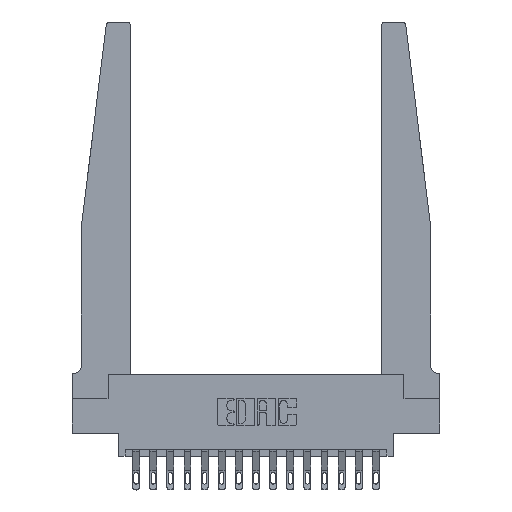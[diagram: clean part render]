
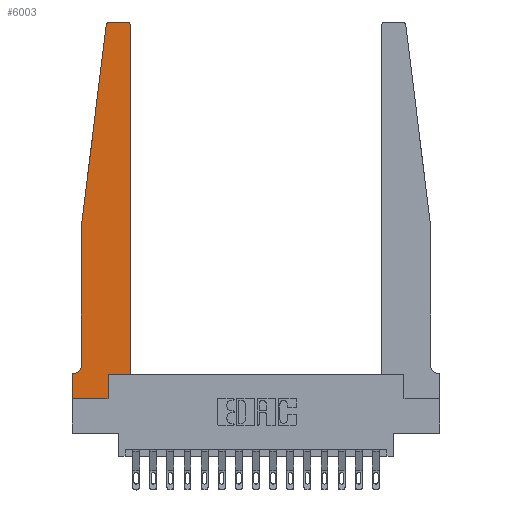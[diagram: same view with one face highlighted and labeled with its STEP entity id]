
A CAD part, top view. The second image highlights one B-rep face of the part: STEP entity #6003.
In plain terms, the highlighted planar face has unit normal (0, 0, 1).
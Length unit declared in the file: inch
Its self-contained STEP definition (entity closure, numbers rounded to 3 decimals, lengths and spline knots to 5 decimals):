
#210 = CARTESIAN_POINT ( 'NONE',  ( 0.425, 0.18, 0.37 ) ) ;
#333 = VECTOR ( 'NONE', #3226, 39.37008 ) ;
#640 = AXIS2_PLACEMENT_3D ( 'NONE', #4934, #15009, #6401 ) ;
#724 = VERTEX_POINT ( 'NONE', #5051 ) ;
#827 = CARTESIAN_POINT ( 'NONE',  ( 0.425, 0.18, 0.37 ) ) ;
#1006 = CARTESIAN_POINT ( 'NONE',  ( 0.27653, 2.75, 0.37 ) ) ;
#1449 = CARTESIAN_POINT ( 'NONE',  ( 0.25, 2.75, 0.37 ) ) ;
#2075 = CARTESIAN_POINT ( 'NONE',  ( 0., 0., 0.37 ) ) ;
#2310 = DIRECTION ( 'NONE',  ( 1., 0., 0. ) ) ;
#2423 = EDGE_CURVE ( 'NONE', #5248, #4190, #13444, .T. ) ;
#2569 = CARTESIAN_POINT ( 'NONE',  ( 0.395, 2.72, 0.37 ) ) ;
#2799 = PLANE ( 'NONE',  #7952 ) ;
#2876 = AXIS2_PLACEMENT_3D ( 'NONE', #2569, #12668, #4031 ) ;
#2906 = LINE ( 'NONE', #6625, #14834 ) ;
#2973 = EDGE_LOOP ( 'NONE', ( #6811, #7140, #7022, #7364, #7803, #7766, #8474, #8508, #8243, #8955, #8969, #13601 ) ) ;
#3065 = LINE ( 'NONE', #827, #10710 ) ;
#3211 = VERTEX_POINT ( 'NONE', #5822 ) ;
#3226 = DIRECTION ( 'NONE',  ( 0., 1., 0. ) ) ;
#3667 = EDGE_CURVE ( 'NONE', #18631, #15239, #2906, .T. ) ;
#3843 = EDGE_CURVE ( 'NONE', #15239, #3211, #15039, .T. ) ;
#4031 = DIRECTION ( 'NONE',  ( 1., 0., 0. ) ) ;
#4035 = CIRCLE ( 'NONE', #640, 0.03 ) ;
#4190 = VERTEX_POINT ( 'NONE', #9826 ) ;
#4252 = DIRECTION ( 'NONE',  ( 1., 0., 0. ) ) ;
#4304 = DIRECTION ( 'NONE',  ( -1., 0., 0. ) ) ;
#4420 = VERTEX_POINT ( 'NONE', #13233 ) ;
#4587 = EDGE_CURVE ( 'NONE', #4783, #18255, #4035, .T. ) ;
#4783 = VERTEX_POINT ( 'NONE', #1006 ) ;
#4934 = CARTESIAN_POINT ( 'NONE',  ( 0.27653, 2.72, 0.37 ) ) ;
#5027 = VERTEX_POINT ( 'NONE', #8942 ) ;
#5051 = CARTESIAN_POINT ( 'NONE',  ( 0.425, 2.72, 0.37 ) ) ;
#5175 = EDGE_CURVE ( 'NONE', #5871, #5248, #10325, .T. ) ;
#5248 = VERTEX_POINT ( 'NONE', #17954 ) ;
#5397 = EDGE_CURVE ( 'NONE', #724, #4420, #17707, .T. ) ;
#5557 = LINE ( 'NONE', #7517, #333 ) ;
#5740 = DIRECTION ( 'NONE',  ( -1., 0., 0. ) ) ;
#5822 = CARTESIAN_POINT ( 'NONE',  ( 0.015, 0.1875, 0.37 ) ) ;
#5871 = VERTEX_POINT ( 'NONE', #12519 ) ;
#6003 = ADVANCED_FACE ( 'NONE', ( #9174 ), #2799, .T. ) ;
#6033 = VECTOR ( 'NONE', #12166, 39.37008 ) ;
#6401 = DIRECTION ( 'NONE',  ( 1., 0., 0. ) ) ;
#6456 = LINE ( 'NONE', #1449, #10309 ) ;
#6591 = AXIS2_PLACEMENT_3D ( 'NONE', #7134, #17171, #8597 ) ;
#6625 = CARTESIAN_POINT ( 'NONE',  ( 0.065, 1.25, 0.37 ) ) ;
#6770 = VERTEX_POINT ( 'NONE', #210 ) ;
#6811 = ORIENTED_EDGE ( 'NONE', *, *, #14784, .T. ) ;
#7022 = ORIENTED_EDGE ( 'NONE', *, *, #17399, .T. ) ;
#7134 = CARTESIAN_POINT ( 'NONE',  ( 0.015, 0.2375, 0.37 ) ) ;
#7140 = ORIENTED_EDGE ( 'NONE', *, *, #4587, .T. ) ;
#7364 = ORIENTED_EDGE ( 'NONE', *, *, #3667, .T. ) ;
#7517 = CARTESIAN_POINT ( 'NONE',  ( 0.425, 0.18, 0.37 ) ) ;
#7766 = ORIENTED_EDGE ( 'NONE', *, *, #9748, .T. ) ;
#7803 = ORIENTED_EDGE ( 'NONE', *, *, #3843, .T. ) ;
#7952 = AXIS2_PLACEMENT_3D ( 'NONE', #17125, #12893, #4252 ) ;
#8243 = ORIENTED_EDGE ( 'NONE', *, *, #2423, .T. ) ;
#8474 = ORIENTED_EDGE ( 'NONE', *, *, #17271, .T. ) ;
#8508 = ORIENTED_EDGE ( 'NONE', *, *, #5175, .T. ) ;
#8597 = DIRECTION ( 'NONE',  ( -1., 0., 0. ) ) ;
#8786 = VECTOR ( 'NONE', #14346, 39.37008 ) ;
#8942 = CARTESIAN_POINT ( 'NONE',  ( 0., 0.1875, 0.37 ) ) ;
#8955 = ORIENTED_EDGE ( 'NONE', *, *, #15739, .T. ) ;
#8969 = ORIENTED_EDGE ( 'NONE', *, *, #14921, .T. ) ;
#9174 = FACE_OUTER_BOUND ( 'NONE', #2973, .T. ) ;
#9459 = CARTESIAN_POINT ( 'NONE',  ( 0.24675, 2.72367, 0.37 ) ) ;
#9748 = EDGE_CURVE ( 'NONE', #3211, #5027, #12185, .T. ) ;
#9826 = CARTESIAN_POINT ( 'NONE',  ( 0.2605, 0.18, 0.37 ) ) ;
#10309 = VECTOR ( 'NONE', #4304, 39.37008 ) ;
#10325 = LINE ( 'NONE', #2075, #6033 ) ;
#10710 = VECTOR ( 'NONE', #2310, 39.37008 ) ;
#11294 = CARTESIAN_POINT ( 'NONE',  ( 0.065, 0.2375, 0.37 ) ) ;
#11410 = DIRECTION ( 'NONE',  ( 0., 1., 0. ) ) ;
#12166 = DIRECTION ( 'NONE',  ( 1., 0., 0. ) ) ;
#12185 = LINE ( 'NONE', #12948, #15520 ) ;
#12519 = CARTESIAN_POINT ( 'NONE',  ( 0., 0., 0.37 ) ) ;
#12668 = DIRECTION ( 'NONE',  ( 0., 0., 1. ) ) ;
#12893 = DIRECTION ( 'NONE',  ( 0., 0., 1. ) ) ;
#12948 = CARTESIAN_POINT ( 'NONE',  ( 0.065, 0.1875, 0.37 ) ) ;
#12969 = CARTESIAN_POINT ( 'NONE',  ( 0., 0., 0.37 ) ) ;
#12993 = VECTOR ( 'NONE', #11410, 39.37008 ) ;
#13218 = DIRECTION ( 'NONE',  ( -0.122, -0.992, 0. ) ) ;
#13233 = CARTESIAN_POINT ( 'NONE',  ( 0.395, 2.75, 0.37 ) ) ;
#13299 = CARTESIAN_POINT ( 'NONE',  ( 0.065, 1.25, 0.37 ) ) ;
#13444 = LINE ( 'NONE', #18523, #12993 ) ;
#13601 = ORIENTED_EDGE ( 'NONE', *, *, #5397, .T. ) ;
#13709 = LINE ( 'NONE', #16054, #17512 ) ;
#13876 = DIRECTION ( 'NONE',  ( 0., -1., 0. ) ) ;
#14346 = DIRECTION ( 'NONE',  ( 0., -1., 0. ) ) ;
#14784 = EDGE_CURVE ( 'NONE', #4420, #4783, #6456, .T. ) ;
#14834 = VECTOR ( 'NONE', #13876, 39.37008 ) ;
#14921 = EDGE_CURVE ( 'NONE', #6770, #724, #5557, .T. ) ;
#15009 = DIRECTION ( 'NONE',  ( 0., 0., 1. ) ) ;
#15037 = LINE ( 'NONE', #12969, #8786 ) ;
#15039 = CIRCLE ( 'NONE', #6591, 0.05 ) ;
#15239 = VERTEX_POINT ( 'NONE', #11294 ) ;
#15520 = VECTOR ( 'NONE', #5740, 39.37008 ) ;
#15739 = EDGE_CURVE ( 'NONE', #4190, #6770, #3065, .T. ) ;
#16054 = CARTESIAN_POINT ( 'NONE',  ( 0.065, 1.25, 0.37 ) ) ;
#17125 = CARTESIAN_POINT ( 'NONE',  ( 0., 0.1875, 0.37 ) ) ;
#17171 = DIRECTION ( 'NONE',  ( 0., 0., -1. ) ) ;
#17271 = EDGE_CURVE ( 'NONE', #5027, #5871, #15037, .T. ) ;
#17399 = EDGE_CURVE ( 'NONE', #18255, #18631, #13709, .T. ) ;
#17512 = VECTOR ( 'NONE', #13218, 39.37008 ) ;
#17707 = CIRCLE ( 'NONE', #2876, 0.03 ) ;
#17954 = CARTESIAN_POINT ( 'NONE',  ( 0.2605, 0., 0.37 ) ) ;
#18255 = VERTEX_POINT ( 'NONE', #9459 ) ;
#18523 = CARTESIAN_POINT ( 'NONE',  ( 0.2605, 0.18, 0.37 ) ) ;
#18631 = VERTEX_POINT ( 'NONE', #13299 ) ;
